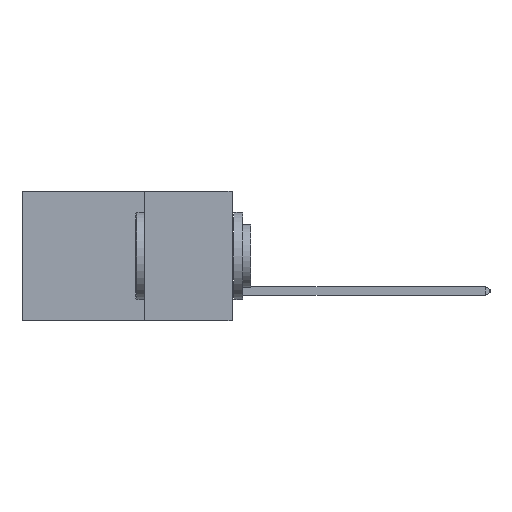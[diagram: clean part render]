
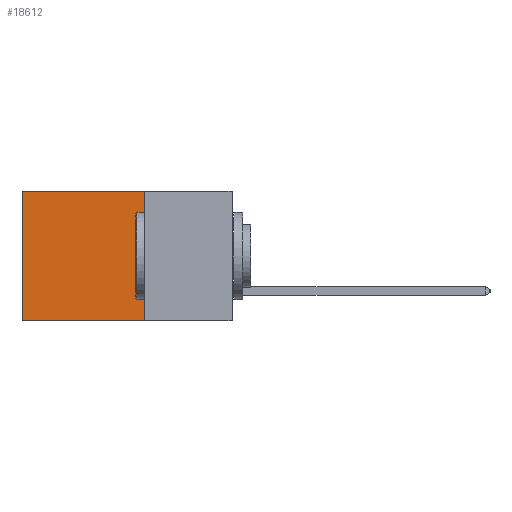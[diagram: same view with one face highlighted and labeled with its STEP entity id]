
A CAD part, left-side view. The second image highlights one B-rep face of the part: STEP entity #18612.
In plain terms, the highlighted planar face has unit normal (-1, 0, 0).
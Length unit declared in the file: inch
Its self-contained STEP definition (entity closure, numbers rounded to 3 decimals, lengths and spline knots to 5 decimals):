
#679 = DIRECTION ( 'NONE',  ( 0., 1., 0. ) ) ;
#846 = EDGE_CURVE ( 'NONE', #1828, #2089, #6788, .T. ) ;
#874 = CARTESIAN_POINT ( 'NONE',  ( 0.2875, 0.25, -0.37 ) ) ;
#954 = CARTESIAN_POINT ( 'NONE',  ( 0.2875, 0.25, -0.37 ) ) ;
#1395 = VERTEX_POINT ( 'NONE', #874 ) ;
#1471 = LINE ( 'NONE', #13335, #10221 ) ;
#1828 = VERTEX_POINT ( 'NONE', #12195 ) ;
#1841 = ORIENTED_EDGE ( 'NONE', *, *, #17466, .F. ) ;
#2089 = VERTEX_POINT ( 'NONE', #5567 ) ;
#2259 = PLANE ( 'NONE',  #4480 ) ;
#2423 = VECTOR ( 'NONE', #13920, 39.37008 ) ;
#3503 = DIRECTION ( 'NONE',  ( 0., 0., -1. ) ) ;
#3913 = DIRECTION ( 'NONE',  ( 0., 0., -1. ) ) ;
#4480 = AXIS2_PLACEMENT_3D ( 'NONE', #12108, #13748, #3913 ) ;
#5359 = EDGE_LOOP ( 'NONE', ( #20417, #1841, #19828, #18170 ) ) ;
#5567 = CARTESIAN_POINT ( 'NONE',  ( 0.2875, 0.6, -0.37 ) ) ;
#6788 = LINE ( 'NONE', #15951, #2423 ) ;
#7560 = DIRECTION ( 'NONE',  ( 0., 1., 0. ) ) ;
#9488 = LINE ( 'NONE', #10530, #14356 ) ;
#9872 = CARTESIAN_POINT ( 'NONE',  ( 0.2875, 0.25, 0. ) ) ;
#9947 = EDGE_CURVE ( 'NONE', #12902, #1828, #9488, .T. ) ;
#10081 = VECTOR ( 'NONE', #7560, 39.37008 ) ;
#10221 = VECTOR ( 'NONE', #3503, 39.37008 ) ;
#10530 = CARTESIAN_POINT ( 'NONE',  ( 0.2875, 0.25, 0. ) ) ;
#12108 = CARTESIAN_POINT ( 'NONE',  ( 0.2875, 0.25, 0. ) ) ;
#12195 = CARTESIAN_POINT ( 'NONE',  ( 0.2875, 0.6, 0. ) ) ;
#12902 = VERTEX_POINT ( 'NONE', #9872 ) ;
#13335 = CARTESIAN_POINT ( 'NONE',  ( 0.2875, 0.25, 0. ) ) ;
#13748 = DIRECTION ( 'NONE',  ( 1., 0., 0. ) ) ;
#13920 = DIRECTION ( 'NONE',  ( 0., 0., -1. ) ) ;
#14356 = VECTOR ( 'NONE', #679, 39.37008 ) ;
#14977 = EDGE_CURVE ( 'NONE', #12902, #1395, #1471, .T. ) ;
#15951 = CARTESIAN_POINT ( 'NONE',  ( 0.2875, 0.6, 0. ) ) ;
#17466 = EDGE_CURVE ( 'NONE', #1395, #2089, #18765, .T. ) ;
#18170 = ORIENTED_EDGE ( 'NONE', *, *, #9947, .T. ) ;
#18243 = FACE_OUTER_BOUND ( 'NONE', #5359, .T. ) ;
#18612 = ADVANCED_FACE ( 'NONE', ( #18243 ), #2259, .F. ) ;
#18765 = LINE ( 'NONE', #954, #10081 ) ;
#19828 = ORIENTED_EDGE ( 'NONE', *, *, #14977, .F. ) ;
#20417 = ORIENTED_EDGE ( 'NONE', *, *, #846, .T. ) ;
